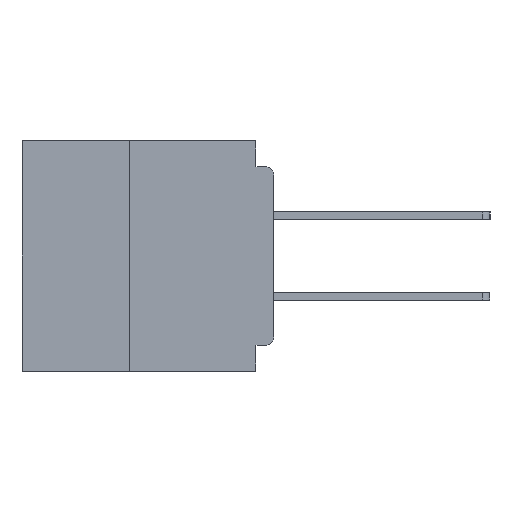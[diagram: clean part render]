
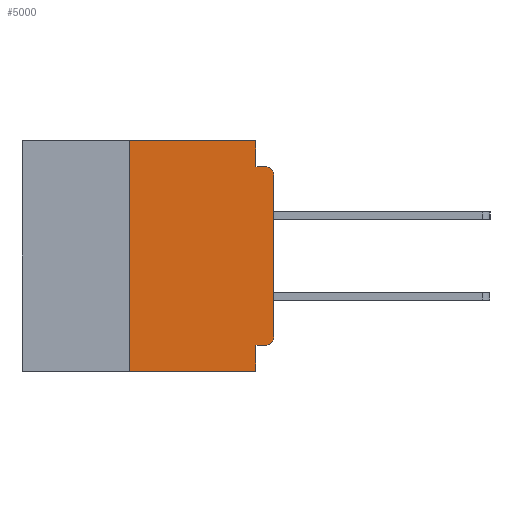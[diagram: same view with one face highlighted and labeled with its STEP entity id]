
A CAD part, left-side view. The second image highlights one B-rep face of the part: STEP entity #5000.
In plain terms, the highlighted planar face has unit normal (-1, 0, 0).
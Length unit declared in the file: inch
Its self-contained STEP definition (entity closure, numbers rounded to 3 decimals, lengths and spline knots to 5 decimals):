
#336 = EDGE_CURVE ( 'NONE', #19706, #8850, #33388, .T. ) ;
#1029 = LINE ( 'NONE', #22109, #35423 ) ;
#1442 = ORIENTED_EDGE ( 'NONE', *, *, #32473, .T. ) ;
#2438 = EDGE_CURVE ( 'NONE', #36925, #33352, #15984, .T. ) ;
#3074 = ORIENTED_EDGE ( 'NONE', *, *, #7227, .F. ) ;
#3764 = VERTEX_POINT ( 'NONE', #17277 ) ;
#4780 = LINE ( 'NONE', #33760, #34223 ) ;
#5000 = ADVANCED_FACE ( 'NONE', ( #30106 ), #30849, .F. ) ;
#5389 = CARTESIAN_POINT ( 'NONE',  ( 0., 0.25, 0. ) ) ;
#5841 = DIRECTION ( 'NONE',  ( -1., 0., 0. ) ) ;
#6533 = VERTEX_POINT ( 'NONE', #6550 ) ;
#6550 = CARTESIAN_POINT ( 'NONE',  ( 0., 0.031, 0. ) ) ;
#7227 = EDGE_CURVE ( 'NONE', #19009, #17603, #35207, .T. ) ;
#7682 = EDGE_CURVE ( 'NONE', #19009, #3764, #28734, .T. ) ;
#8850 = VERTEX_POINT ( 'NONE', #20275 ) ;
#8919 = ORIENTED_EDGE ( 'NONE', *, *, #336, .T. ) ;
#9654 = ORIENTED_EDGE ( 'NONE', *, *, #26611, .F. ) ;
#10574 = DIRECTION ( 'NONE',  ( 0., 0., 1. ) ) ;
#10934 = EDGE_LOOP ( 'NONE', ( #1442, #18963, #14293, #9654, #23521, #19157, #8919, #12544, #3074, #11757 ) ) ;
#11615 = VECTOR ( 'NONE', #12931, 39.37008 ) ;
#11757 = ORIENTED_EDGE ( 'NONE', *, *, #7682, .T. ) ;
#12544 = ORIENTED_EDGE ( 'NONE', *, *, #18357, .F. ) ;
#12557 = EDGE_CURVE ( 'NONE', #17752, #6533, #32470, .T. ) ;
#12931 = DIRECTION ( 'NONE',  ( 0., 0., -1. ) ) ;
#14293 = ORIENTED_EDGE ( 'NONE', *, *, #2438, .F. ) ;
#15158 = AXIS2_PLACEMENT_3D ( 'NONE', #23099, #5841, #25938 ) ;
#15177 = CARTESIAN_POINT ( 'NONE',  ( 0., 0.437, 0. ) ) ;
#15553 = VECTOR ( 'NONE', #24470, 39.37008 ) ;
#15984 = LINE ( 'NONE', #25205, #15553 ) ;
#16386 = CARTESIAN_POINT ( 'NONE',  ( 0., 0., 0. ) ) ;
#17132 = CARTESIAN_POINT ( 'NONE',  ( 0., 0.015, -0.06 ) ) ;
#17277 = CARTESIAN_POINT ( 'NONE',  ( 0., 0., -0.34 ) ) ;
#17603 = VERTEX_POINT ( 'NONE', #35990 ) ;
#17752 = VERTEX_POINT ( 'NONE', #5389 ) ;
#18268 = DIRECTION ( 'NONE',  ( 0., 1., 0. ) ) ;
#18357 = EDGE_CURVE ( 'NONE', #17603, #8850, #4780, .T. ) ;
#18374 = VECTOR ( 'NONE', #21533, 39.37008 ) ;
#18542 = CIRCLE ( 'NONE', #36203, 0.015 ) ;
#18946 = CARTESIAN_POINT ( 'NONE',  ( 0., 0.031, -0.045 ) ) ;
#18963 = ORIENTED_EDGE ( 'NONE', *, *, #33563, .T. ) ;
#19009 = VERTEX_POINT ( 'NONE', #30981 ) ;
#19090 = VECTOR ( 'NONE', #10574, 39.37008 ) ;
#19157 = ORIENTED_EDGE ( 'NONE', *, *, #24269, .F. ) ;
#19706 = VERTEX_POINT ( 'NONE', #29094 ) ;
#19993 = DIRECTION ( 'NONE',  ( 0., 0., -1. ) ) ;
#20156 = LINE ( 'NONE', #32792, #11615 ) ;
#20275 = CARTESIAN_POINT ( 'NONE',  ( 0., 0.031, -0.4 ) ) ;
#20854 = LINE ( 'NONE', #16386, #19090 ) ;
#21411 = CARTESIAN_POINT ( 'NONE',  ( 0., 0.437, -0.4 ) ) ;
#21533 = DIRECTION ( 'NONE',  ( 0., -1., 0. ) ) ;
#21906 = CARTESIAN_POINT ( 'NONE',  ( 0., 0.015, -0.045 ) ) ;
#22109 = CARTESIAN_POINT ( 'NONE',  ( 0., 0.25, -0.4 ) ) ;
#23099 = CARTESIAN_POINT ( 'NONE',  ( 0., 0.015, -0.34 ) ) ;
#23521 = ORIENTED_EDGE ( 'NONE', *, *, #12557, .F. ) ;
#24099 = VECTOR ( 'NONE', #32319, 39.37008 ) ;
#24269 = EDGE_CURVE ( 'NONE', #19706, #17752, #1029, .T. ) ;
#24470 = DIRECTION ( 'NONE',  ( 0., -1., 0. ) ) ;
#25205 = CARTESIAN_POINT ( 'NONE',  ( 0., 0., -0.045 ) ) ;
#25683 = VERTEX_POINT ( 'NONE', #28603 ) ;
#25938 = DIRECTION ( 'NONE',  ( 0., 0., -1. ) ) ;
#26611 = EDGE_CURVE ( 'NONE', #6533, #36925, #20156, .T. ) ;
#27893 = VECTOR ( 'NONE', #18268, 39.37008 ) ;
#28603 = CARTESIAN_POINT ( 'NONE',  ( 0., 0., -0.06 ) ) ;
#28734 = CIRCLE ( 'NONE', #15158, 0.015 ) ;
#29094 = CARTESIAN_POINT ( 'NONE',  ( 0., 0.25, -0.4 ) ) ;
#30106 = FACE_OUTER_BOUND ( 'NONE', #10934, .T. ) ;
#30673 = DIRECTION ( 'NONE',  ( 0., 0., 1. ) ) ;
#30734 = DIRECTION ( 'NONE',  ( 0., 0., -1. ) ) ;
#30763 = DIRECTION ( 'NONE',  ( 1., 0., 0. ) ) ;
#30849 = PLANE ( 'NONE',  #31111 ) ;
#30981 = CARTESIAN_POINT ( 'NONE',  ( 0., 0.015, -0.355 ) ) ;
#31111 = AXIS2_PLACEMENT_3D ( 'NONE', #31430, #30763, #30734 ) ;
#31430 = CARTESIAN_POINT ( 'NONE',  ( 0., 0.437, 0. ) ) ;
#32319 = DIRECTION ( 'NONE',  ( 0., -1., 0. ) ) ;
#32364 = CARTESIAN_POINT ( 'NONE',  ( 0., 0., -0.355 ) ) ;
#32470 = LINE ( 'NONE', #15177, #24099 ) ;
#32473 = EDGE_CURVE ( 'NONE', #3764, #25683, #20854, .T. ) ;
#32792 = CARTESIAN_POINT ( 'NONE',  ( 0., 0.031, 0. ) ) ;
#33352 = VERTEX_POINT ( 'NONE', #21906 ) ;
#33388 = LINE ( 'NONE', #21411, #18374 ) ;
#33563 = EDGE_CURVE ( 'NONE', #25683, #33352, #18542, .T. ) ;
#33760 = CARTESIAN_POINT ( 'NONE',  ( 0., 0.031, -0.4 ) ) ;
#34223 = VECTOR ( 'NONE', #36463, 39.37008 ) ;
#35207 = LINE ( 'NONE', #32364, #27893 ) ;
#35423 = VECTOR ( 'NONE', #30673, 39.37008 ) ;
#35990 = CARTESIAN_POINT ( 'NONE',  ( 0., 0.031, -0.355 ) ) ;
#36203 = AXIS2_PLACEMENT_3D ( 'NONE', #17132, #36723, #19993 ) ;
#36463 = DIRECTION ( 'NONE',  ( 0., 0., -1. ) ) ;
#36723 = DIRECTION ( 'NONE',  ( -1., 0., 0. ) ) ;
#36925 = VERTEX_POINT ( 'NONE', #18946 ) ;
